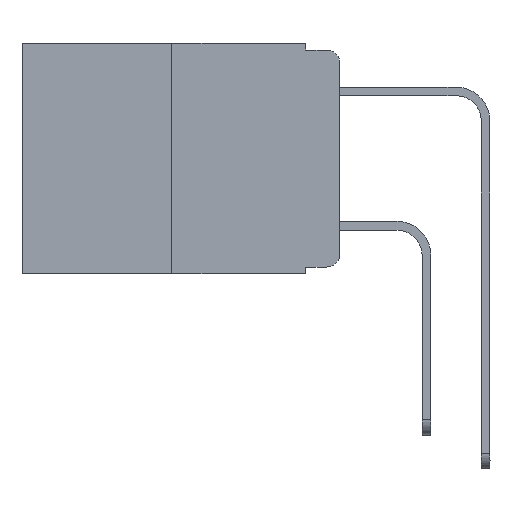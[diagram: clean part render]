
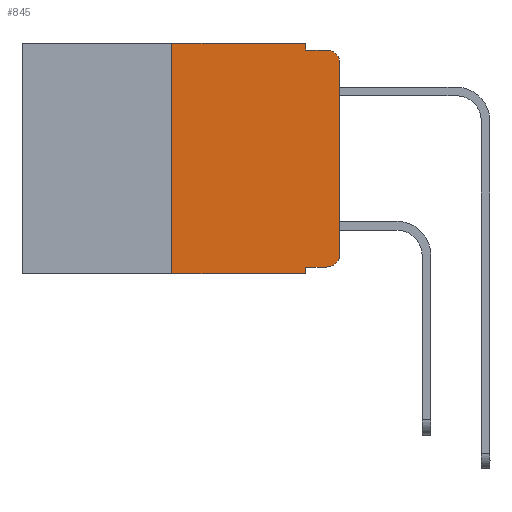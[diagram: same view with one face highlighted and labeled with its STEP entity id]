
A CAD part, left-side view. The second image highlights one B-rep face of the part: STEP entity #845.
In plain terms, the highlighted planar face has unit normal (-1, 0, 0).
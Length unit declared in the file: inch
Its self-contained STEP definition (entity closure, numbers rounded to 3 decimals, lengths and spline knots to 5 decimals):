
#390 = DIRECTION ( 'NONE',  ( 1., 0., 0. ) ) ;
#845 = ADVANCED_FACE ( 'NONE', ( #12363 ), #6383, .F. ) ;
#846 = CARTESIAN_POINT ( 'NONE',  ( 0., 0., -0.313 ) ) ;
#1722 = LINE ( 'NONE', #23997, #7450 ) ;
#1742 = VECTOR ( 'NONE', #19391, 39.37008 ) ;
#2325 = LINE ( 'NONE', #26077, #25426 ) ;
#2726 = ORIENTED_EDGE ( 'NONE', *, *, #4137, .F. ) ;
#3231 = CARTESIAN_POINT ( 'NONE',  ( 0., 0.051, 0. ) ) ;
#3387 = CIRCLE ( 'NONE', #15227, 0.02 ) ;
#3948 = CARTESIAN_POINT ( 'NONE',  ( 0., 0., 0. ) ) ;
#4137 = EDGE_CURVE ( 'NONE', #20156, #16779, #2325, .T. ) ;
#4397 = EDGE_CURVE ( 'NONE', #5056, #17629, #21655, .T. ) ;
#4483 = ORIENTED_EDGE ( 'NONE', *, *, #4397, .F. ) ;
#5056 = VERTEX_POINT ( 'NONE', #11970 ) ;
#5069 = DIRECTION ( 'NONE',  ( 0., 0., -1. ) ) ;
#5243 = CARTESIAN_POINT ( 'NONE',  ( 0., 0.051, -0.01 ) ) ;
#5674 = CARTESIAN_POINT ( 'NONE',  ( 0., 0.25, -0.343 ) ) ;
#5719 = EDGE_CURVE ( 'NONE', #24708, #7755, #9974, .T. ) ;
#5922 = EDGE_LOOP ( 'NONE', ( #14307, #12625, #4483, #14265, #11054, #2726, #12714, #21652, #18980, #7521 ) ) ;
#6083 = LINE ( 'NONE', #3948, #15269 ) ;
#6108 = DIRECTION ( 'NONE',  ( 0., -1., 0. ) ) ;
#6383 = PLANE ( 'NONE',  #24022 ) ;
#6534 = VERTEX_POINT ( 'NONE', #21072 ) ;
#7061 = VERTEX_POINT ( 'NONE', #13041 ) ;
#7352 = CARTESIAN_POINT ( 'NONE',  ( 0., 0.02, -0.03 ) ) ;
#7450 = VECTOR ( 'NONE', #6108, 39.37008 ) ;
#7521 = ORIENTED_EDGE ( 'NONE', *, *, #5719, .T. ) ;
#7713 = VECTOR ( 'NONE', #13327, 39.37008 ) ;
#7755 = VERTEX_POINT ( 'NONE', #846 ) ;
#7861 = EDGE_CURVE ( 'NONE', #16779, #6534, #12817, .T. ) ;
#7966 = CARTESIAN_POINT ( 'NONE',  ( 0., 0., -0.03 ) ) ;
#8513 = DIRECTION ( 'NONE',  ( 0., 0., -1. ) ) ;
#8892 = CARTESIAN_POINT ( 'NONE',  ( 0., 0.25, 0. ) ) ;
#9016 = VERTEX_POINT ( 'NONE', #7966 ) ;
#9054 = CARTESIAN_POINT ( 'NONE',  ( 0., 0.051, 0. ) ) ;
#9114 = CARTESIAN_POINT ( 'NONE',  ( 0., 0.02, -0.333 ) ) ;
#9974 = CIRCLE ( 'NONE', #18435, 0.02 ) ;
#10949 = DIRECTION ( 'NONE',  ( 0., 0., -1. ) ) ;
#11054 = ORIENTED_EDGE ( 'NONE', *, *, #7861, .F. ) ;
#11790 = DIRECTION ( 'NONE',  ( 0., -1., 0. ) ) ;
#11970 = CARTESIAN_POINT ( 'NONE',  ( 0., 0.051, -0.01 ) ) ;
#12363 = FACE_OUTER_BOUND ( 'NONE', #5922, .T. ) ;
#12625 = ORIENTED_EDGE ( 'NONE', *, *, #13423, .T. ) ;
#12714 = ORIENTED_EDGE ( 'NONE', *, *, #25628, .T. ) ;
#12817 = LINE ( 'NONE', #20739, #23100 ) ;
#13041 = CARTESIAN_POINT ( 'NONE',  ( 0., 0.051, -0.343 ) ) ;
#13258 = CARTESIAN_POINT ( 'NONE',  ( 0., 0.473, -0.343 ) ) ;
#13327 = DIRECTION ( 'NONE',  ( 0., -1., 0. ) ) ;
#13423 = EDGE_CURVE ( 'NONE', #9016, #17629, #3387, .T. ) ;
#14265 = ORIENTED_EDGE ( 'NONE', *, *, #17916, .F. ) ;
#14307 = ORIENTED_EDGE ( 'NONE', *, *, #14654, .T. ) ;
#14654 = EDGE_CURVE ( 'NONE', #7755, #9016, #6083, .T. ) ;
#15134 = LINE ( 'NONE', #9054, #19545 ) ;
#15158 = DIRECTION ( 'NONE',  ( 0., 0., -1. ) ) ;
#15227 = AXIS2_PLACEMENT_3D ( 'NONE', #7352, #19261, #15158 ) ;
#15269 = VECTOR ( 'NONE', #16662, 39.37008 ) ;
#15270 = EDGE_CURVE ( 'NONE', #20286, #7061, #15134, .T. ) ;
#16353 = VECTOR ( 'NONE', #11790, 39.37008 ) ;
#16407 = CARTESIAN_POINT ( 'NONE',  ( 0., 0.051, -0.333 ) ) ;
#16507 = CARTESIAN_POINT ( 'NONE',  ( 0., 0.02, -0.01 ) ) ;
#16662 = DIRECTION ( 'NONE',  ( 0., 0., 1. ) ) ;
#16779 = VERTEX_POINT ( 'NONE', #8892 ) ;
#17629 = VERTEX_POINT ( 'NONE', #16507 ) ;
#17916 = EDGE_CURVE ( 'NONE', #6534, #5056, #23507, .T. ) ;
#18435 = AXIS2_PLACEMENT_3D ( 'NONE', #20874, #24998, #10949 ) ;
#18980 = ORIENTED_EDGE ( 'NONE', *, *, #23909, .T. ) ;
#19261 = DIRECTION ( 'NONE',  ( -1., 0., 0. ) ) ;
#19391 = DIRECTION ( 'NONE',  ( 0., 0., -1. ) ) ;
#19545 = VECTOR ( 'NONE', #5069, 39.37008 ) ;
#20156 = VERTEX_POINT ( 'NONE', #5674 ) ;
#20286 = VERTEX_POINT ( 'NONE', #16407 ) ;
#20739 = CARTESIAN_POINT ( 'NONE',  ( 0., 0.473, 0. ) ) ;
#20874 = CARTESIAN_POINT ( 'NONE',  ( 0., 0.02, -0.313 ) ) ;
#21072 = CARTESIAN_POINT ( 'NONE',  ( 0., 0.051, 0. ) ) ;
#21652 = ORIENTED_EDGE ( 'NONE', *, *, #15270, .F. ) ;
#21655 = LINE ( 'NONE', #5243, #7713 ) ;
#22083 = DIRECTION ( 'NONE',  ( 0., 0., 1. ) ) ;
#22538 = CARTESIAN_POINT ( 'NONE',  ( 0., 0.473, 0. ) ) ;
#22735 = DIRECTION ( 'NONE',  ( 0., -1., 0. ) ) ;
#23100 = VECTOR ( 'NONE', #22735, 39.37008 ) ;
#23507 = LINE ( 'NONE', #3231, #1742 ) ;
#23836 = LINE ( 'NONE', #13258, #16353 ) ;
#23909 = EDGE_CURVE ( 'NONE', #20286, #24708, #1722, .T. ) ;
#23997 = CARTESIAN_POINT ( 'NONE',  ( 0., 0.051, -0.333 ) ) ;
#24022 = AXIS2_PLACEMENT_3D ( 'NONE', #22538, #390, #8513 ) ;
#24708 = VERTEX_POINT ( 'NONE', #9114 ) ;
#24998 = DIRECTION ( 'NONE',  ( -1., 0., 0. ) ) ;
#25426 = VECTOR ( 'NONE', #22083, 39.37008 ) ;
#25628 = EDGE_CURVE ( 'NONE', #20156, #7061, #23836, .T. ) ;
#26077 = CARTESIAN_POINT ( 'NONE',  ( 0., 0.25, 0. ) ) ;
